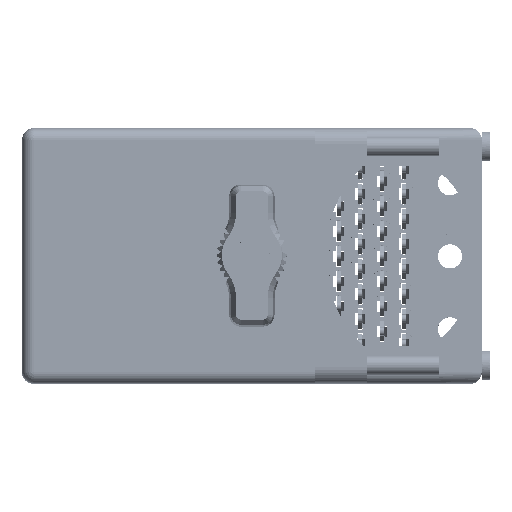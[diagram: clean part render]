
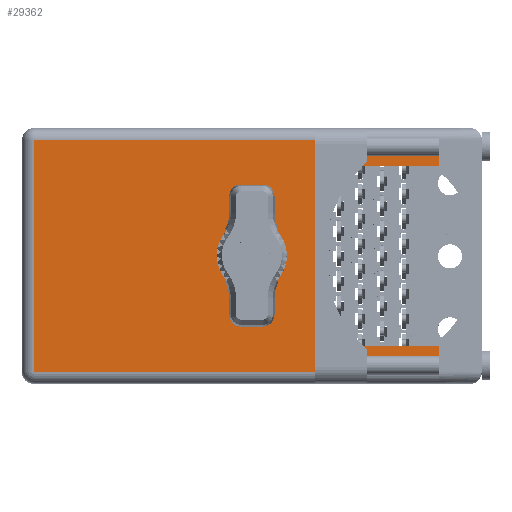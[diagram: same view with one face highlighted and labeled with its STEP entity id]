
A CAD part, top view. The second image highlights one B-rep face of the part: STEP entity #29362.
In plain terms, the highlighted face is planar.
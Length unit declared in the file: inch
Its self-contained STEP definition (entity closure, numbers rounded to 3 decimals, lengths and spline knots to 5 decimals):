
#1169 = CARTESIAN_POINT ( 'NONE',  ( 2.499, 2.03, -1.305 ) ) ;
#2707 = ORIENTED_EDGE ( 'NONE', *, *, #96369, .T. ) ;
#3104 = CARTESIAN_POINT ( 'NONE',  ( 2.499, 2.03, -1.46 ) ) ;
#5892 = AXIS2_PLACEMENT_3D ( 'NONE', #55483, #20464, #106348 ) ;
#6665 = CARTESIAN_POINT ( 'NONE',  ( 1.3775, 2.03, -0.765 ) ) ;
#7505 = DIRECTION ( 'NONE',  ( 0., 1., 0. ) ) ;
#8340 = DIRECTION ( 'NONE',  ( 0., 0., 1. ) ) ;
#9684 = DIRECTION ( 'NONE',  ( 1., 0., 0. ) ) ;
#9857 = EDGE_CURVE ( 'NONE', #14991, #85321, #97169, .T. ) ;
#10160 = LINE ( 'NONE', #77080, #16819 ) ;
#10170 = LINE ( 'NONE', #18469, #15580 ) ;
#14991 = VERTEX_POINT ( 'NONE', #69408 ) ;
#15580 = VECTOR ( 'NONE', #93697, 39.37008 ) ;
#15909 = VECTOR ( 'NONE', #90865, 39.37008 ) ;
#16819 = VECTOR ( 'NONE', #18376, 39.37008 ) ;
#18003 = CARTESIAN_POINT ( 'NONE',  ( 2.499, 2.03, -0.07 ) ) ;
#18376 = DIRECTION ( 'NONE',  ( -1., 0., 0. ) ) ;
#18469 = CARTESIAN_POINT ( 'NONE',  ( 2.499, 2.03, -1.53 ) ) ;
#18907 = ORIENTED_EDGE ( 'NONE', *, *, #24683, .T. ) ;
#20464 = DIRECTION ( 'NONE',  ( 0., 1., 0. ) ) ;
#21853 = VERTEX_POINT ( 'NONE', #62126 ) ;
#22167 = CARTESIAN_POINT ( 'NONE',  ( 1.3775, 2.03, -0.935 ) ) ;
#23971 = DIRECTION ( 'NONE',  ( 0., 0., 1. ) ) ;
#24683 = EDGE_CURVE ( 'NONE', #101573, #21853, #76732, .T. ) ;
#25059 = ORIENTED_EDGE ( 'NONE', *, *, #37645, .T. ) ;
#26644 = AXIS2_PLACEMENT_3D ( 'NONE', #6665, #90367, #23971 ) ;
#29362 = ADVANCED_FACE ( 'NONE', ( #85065, #74508 ), #75051, .T. ) ;
#29575 = CARTESIAN_POINT ( 'NONE',  ( 1.785, 2.03, -1.305 ) ) ;
#30888 = ORIENTED_EDGE ( 'NONE', *, *, #31666, .F. ) ;
#31666 = EDGE_CURVE ( 'NONE', #50190, #79182, #76760, .T. ) ;
#33077 = CARTESIAN_POINT ( 'NONE',  ( 1.785, 2.03, -1.305 ) ) ;
#33132 = ORIENTED_EDGE ( 'NONE', *, *, #61369, .F. ) ;
#36911 = CARTESIAN_POINT ( 'NONE',  ( 2.499, 2.03, -1.53 ) ) ;
#37645 = EDGE_CURVE ( 'NONE', #55503, #14991, #10160, .T. ) ;
#41596 = CIRCLE ( 'NONE', #5892, 0.17 ) ;
#46984 = AXIS2_PLACEMENT_3D ( 'NONE', #65836, #7505, #48842 ) ;
#48218 = LINE ( 'NONE', #36911, #71909 ) ;
#48842 = DIRECTION ( 'NONE',  ( 0., 0., 1. ) ) ;
#50043 = CARTESIAN_POINT ( 'NONE',  ( 0.07, 2.03, -1.53 ) ) ;
#50190 = VERTEX_POINT ( 'NONE', #22167 ) ;
#50915 = VERTEX_POINT ( 'NONE', #56676 ) ;
#51541 = CARTESIAN_POINT ( 'NONE',  ( 0.07, 2.03, -0.07 ) ) ;
#52340 = VECTOR ( 'NONE', #8340, 39.37008 ) ;
#54693 = VECTOR ( 'NONE', #100873, 39.37008 ) ;
#55483 = CARTESIAN_POINT ( 'NONE',  ( 1.3775, 2.03, -0.765 ) ) ;
#55503 = VERTEX_POINT ( 'NONE', #3104 ) ;
#55615 = EDGE_CURVE ( 'NONE', #79182, #50190, #41596, .T. ) ;
#56676 = CARTESIAN_POINT ( 'NONE',  ( 2.499, 2.03, -1.305 ) ) ;
#60786 = DIRECTION ( 'NONE',  ( 1., 0., 0. ) ) ;
#61369 = EDGE_CURVE ( 'NONE', #55503, #50915, #10170, .T. ) ;
#62126 = CARTESIAN_POINT ( 'NONE',  ( 1.785, 2.03, -0.225 ) ) ;
#62659 = DIRECTION ( 'NONE',  ( 0., 0., 1. ) ) ;
#63226 = ORIENTED_EDGE ( 'NONE', *, *, #55615, .F. ) ;
#65836 = CARTESIAN_POINT ( 'NONE',  ( 0., 2.03, -1.53 ) ) ;
#66290 = ORIENTED_EDGE ( 'NONE', *, *, #97090, .F. ) ;
#69408 = CARTESIAN_POINT ( 'NONE',  ( 0.07, 2.03, -1.46 ) ) ;
#71909 = VECTOR ( 'NONE', #62659, 39.37008 ) ;
#73046 = CARTESIAN_POINT ( 'NONE',  ( 2.499, 2.03, -0.225 ) ) ;
#73470 = VECTOR ( 'NONE', #60786, 39.37008 ) ;
#74508 = FACE_BOUND ( 'NONE', #79863, .T. ) ;
#74563 = CARTESIAN_POINT ( 'NONE',  ( 2.499, 2.03, -0.07 ) ) ;
#74826 = VECTOR ( 'NONE', #9684, 39.37008 ) ;
#75051 = PLANE ( 'NONE',  #46984 ) ;
#75811 = ORIENTED_EDGE ( 'NONE', *, *, #9857, .T. ) ;
#76036 = ORIENTED_EDGE ( 'NONE', *, *, #98561, .T. ) ;
#76732 = LINE ( 'NONE', #91963, #15909 ) ;
#76760 = CIRCLE ( 'NONE', #26644, 0.17 ) ;
#77080 = CARTESIAN_POINT ( 'NONE',  ( 0., 2.03, -1.46 ) ) ;
#79182 = VERTEX_POINT ( 'NONE', #104523 ) ;
#79863 = EDGE_LOOP ( 'NONE', ( #63226, #30888 ) ) ;
#83402 = VERTEX_POINT ( 'NONE', #29575 ) ;
#84009 = LINE ( 'NONE', #1169, #74826 ) ;
#85065 = FACE_OUTER_BOUND ( 'NONE', #87367, .T. ) ;
#85321 = VERTEX_POINT ( 'NONE', #51541 ) ;
#86472 = EDGE_CURVE ( 'NONE', #85321, #94871, #109130, .T. ) ;
#87367 = EDGE_LOOP ( 'NONE', ( #75811, #106338, #66290, #18907, #76036, #2707, #33132, #25059 ) ) ;
#90367 = DIRECTION ( 'NONE',  ( 0., 1., 0. ) ) ;
#90865 = DIRECTION ( 'NONE',  ( -1., 0., 0. ) ) ;
#91963 = CARTESIAN_POINT ( 'NONE',  ( 2.499, 2.03, -0.225 ) ) ;
#93697 = DIRECTION ( 'NONE',  ( 0., 0., 1. ) ) ;
#94871 = VERTEX_POINT ( 'NONE', #74563 ) ;
#96369 = EDGE_CURVE ( 'NONE', #83402, #50915, #84009, .T. ) ;
#96892 = LINE ( 'NONE', #33077, #54693 ) ;
#97090 = EDGE_CURVE ( 'NONE', #101573, #94871, #48218, .T. ) ;
#97169 = LINE ( 'NONE', #50043, #52340 ) ;
#98561 = EDGE_CURVE ( 'NONE', #21853, #83402, #96892, .T. ) ;
#100873 = DIRECTION ( 'NONE',  ( 0., 0., -1. ) ) ;
#101573 = VERTEX_POINT ( 'NONE', #73046 ) ;
#104523 = CARTESIAN_POINT ( 'NONE',  ( 1.3775, 2.03, -0.595 ) ) ;
#106338 = ORIENTED_EDGE ( 'NONE', *, *, #86472, .T. ) ;
#106348 = DIRECTION ( 'NONE',  ( 0., 0., 1. ) ) ;
#109130 = LINE ( 'NONE', #18003, #73470 ) ;
